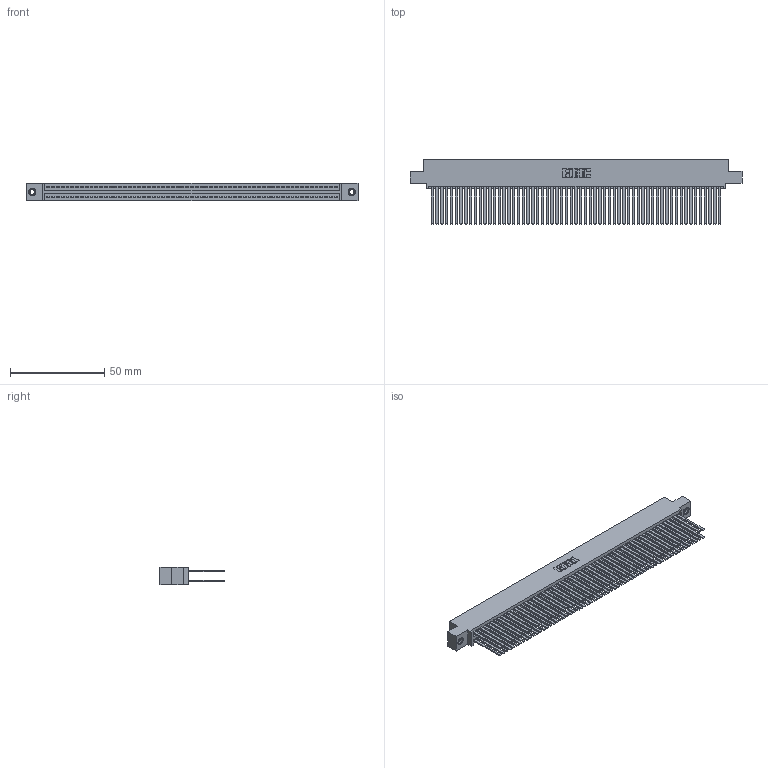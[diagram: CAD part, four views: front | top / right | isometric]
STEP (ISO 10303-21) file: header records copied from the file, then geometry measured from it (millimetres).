
FILE_DESCRIPTION (( 'STEP AP203' ), '1' );
FILE_NAME ('395-122-544-507.STEP', '2018-12-03T19:17:03', ( '' ), ( '' ), 'SwSTEP 2.0', 'SolidWorks 2016', '' );
FILE_SCHEMA (( 'CONFIG_CONTROL_DESIGN' ));
Products named in the file (4): 345-250-001_345-250-005-103; 345-292-001_345-293-144; 345 Part_0.110 Offset - 0.156 Dia-TI; 395-122-544-507
Assembly tree (125 placements, depth 2):
  395-122-544-507
    345 Part_0.110 Offset - 0.156 Dia-TI
    345-292-001_345-293-144  x122
    345-250-001_345-250-005-103  x2
Bounding box: 176.15 x 33.96 x 9.4 mm (x, y, z)
Volume: 18911 mm3; surface area: 33454.8 mm2
Topology: 125 solids, 125 shells, 5558 faces, 16471 edges, 10810 vertices
Faces by surface type: plane 3654, cylinder 1888, cone 12, torus 4
Entity records: 46438 total; most frequent: CARTESIAN_POINT 7747, ORIENTED_EDGE 7674, DIRECTION 6831, EDGE_CURVE 3837, VECTOR 3445, LINE 3445, VERTEX_POINT 2552, AXIS2_PLACEMENT_3D 1693
